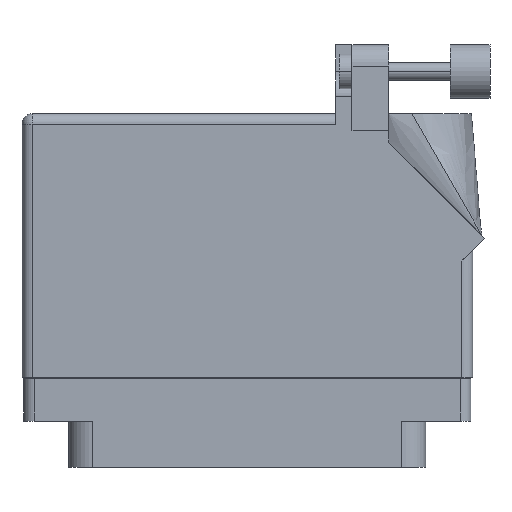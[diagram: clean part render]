
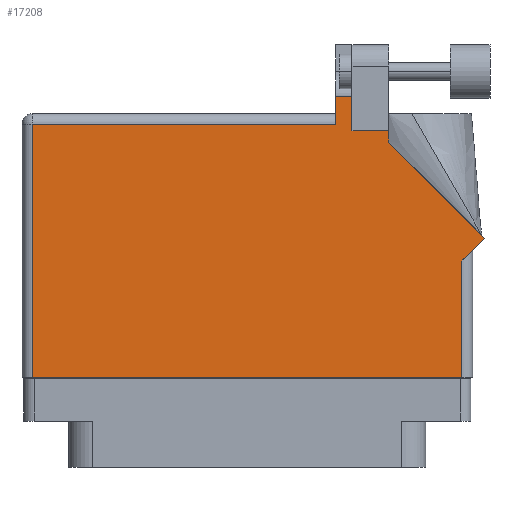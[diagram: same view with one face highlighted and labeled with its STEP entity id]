
A CAD part, front view. The second image highlights one B-rep face of the part: STEP entity #17208.
In plain terms, the highlighted face is planar.
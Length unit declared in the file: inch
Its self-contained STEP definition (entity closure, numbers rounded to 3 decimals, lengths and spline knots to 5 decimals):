
#49 = CARTESIAN_POINT ( 'NONE',  ( 0.513, 1.5315, 0.455 ) ) ;
#221 = VECTOR ( 'NONE', #23083, 39.37008 ) ;
#785 = DIRECTION ( 'NONE',  ( -0.707, 0.707, 0. ) ) ;
#1640 = VERTEX_POINT ( 'NONE', #49 ) ;
#1828 = CARTESIAN_POINT ( 'NONE',  ( 0.82, 1.26442, 0.455 ) ) ;
#2082 = CARTESIAN_POINT ( 'NONE',  ( 0.607, 1.33, 0.455 ) ) ;
#2425 = CARTESIAN_POINT ( 'NONE',  ( 1.244, 0.575, 0.455 ) ) ;
#2976 = DIRECTION ( 'NONE',  ( 0., 1., 0. ) ) ;
#3350 = LINE ( 'NONE', #6694, #26731 ) ;
#3666 = LINE ( 'NONE', #47013, #47791 ) ;
#3968 = CARTESIAN_POINT ( 'NONE',  ( -1.306, -0.1, 0.455 ) ) ;
#4143 = DIRECTION ( 'NONE',  ( 1., 0., 0. ) ) ;
#5109 = DIRECTION ( 'NONE',  ( -1., 0., 0. ) ) ;
#5565 = CARTESIAN_POINT ( 'NONE',  ( 0.82, 1.26442, 0.455 ) ) ;
#5858 = CARTESIAN_POINT ( 'NONE',  ( 0.82, 1.33, 0.455 ) ) ;
#6465 = FACE_OUTER_BOUND ( 'NONE', #18573, .T. ) ;
#6694 = CARTESIAN_POINT ( 'NONE',  ( 0.93777, 1.5315, 0.455 ) ) ;
#7440 = LINE ( 'NONE', #3968, #37716 ) ;
#7619 = LINE ( 'NONE', #27489, #15826 ) ;
#8244 = ORIENTED_EDGE ( 'NONE', *, *, #24293, .T. ) ;
#8708 = DIRECTION ( 'NONE',  ( -1., 0., 0. ) ) ;
#8728 = CARTESIAN_POINT ( 'NONE',  ( -1.306, 1.368, 0.455 ) ) ;
#8995 = LINE ( 'NONE', #29509, #38632 ) ;
#9970 = VERTEX_POINT ( 'NONE', #2425 ) ;
#10563 = VERTEX_POINT ( 'NONE', #39279 ) ;
#10873 = AXIS2_PLACEMENT_3D ( 'NONE', #33602, #33244, #8708 ) ;
#11435 = VERTEX_POINT ( 'NONE', #23367 ) ;
#11550 = DIRECTION ( 'NONE',  ( 0., -1., 0. ) ) ;
#12171 = LINE ( 'NONE', #31360, #221 ) ;
#12985 = VECTOR ( 'NONE', #41783, 39.37008 ) ;
#14093 = EDGE_CURVE ( 'NONE', #51600, #27255, #48488, .T. ) ;
#14761 = EDGE_CURVE ( 'NONE', #37501, #10563, #7440, .T. ) ;
#15752 = CARTESIAN_POINT ( 'NONE',  ( -1.244, -0.1, 0.455 ) ) ;
#15826 = VECTOR ( 'NONE', #2976, 39.37008 ) ;
#17208 = ADVANCED_FACE ( 'NONE', ( #6465 ), #21335, .F. ) ;
#18041 = DIRECTION ( 'NONE',  ( 0., 1., 0. ) ) ;
#18573 = EDGE_LOOP ( 'NONE', ( #34944, #49988, #47823, #34438, #8244, #42310, #28356, #40156, #36596, #33503, #45584 ) ) ;
#18603 = CARTESIAN_POINT ( 'NONE',  ( -1.244, 1.368, 0.455 ) ) ;
#21335 = PLANE ( 'NONE',  #10873 ) ;
#22110 = EDGE_CURVE ( 'NONE', #22245, #1640, #3350, .T. ) ;
#22241 = VECTOR ( 'NONE', #47066, 39.37008 ) ;
#22245 = VERTEX_POINT ( 'NONE', #40136 ) ;
#22596 = LINE ( 'NONE', #43610, #27086 ) ;
#23083 = DIRECTION ( 'NONE',  ( 0.707, 0.707, 0. ) ) ;
#23367 = CARTESIAN_POINT ( 'NONE',  ( 0.513, 1.368, 0.455 ) ) ;
#23704 = LINE ( 'NONE', #5858, #12985 ) ;
#24293 = EDGE_CURVE ( 'NONE', #24915, #37501, #22596, .T. ) ;
#24915 = VERTEX_POINT ( 'NONE', #18603 ) ;
#26731 = VECTOR ( 'NONE', #5109, 39.37008 ) ;
#27063 = VECTOR ( 'NONE', #18041, 39.37008 ) ;
#27086 = VECTOR ( 'NONE', #11550, 39.37008 ) ;
#27255 = VERTEX_POINT ( 'NONE', #47784 ) ;
#27489 = CARTESIAN_POINT ( 'NONE',  ( 0.607, 1.33, 0.455 ) ) ;
#27803 = EDGE_CURVE ( 'NONE', #10563, #9970, #33027, .T. ) ;
#28356 = ORIENTED_EDGE ( 'NONE', *, *, #27803, .T. ) ;
#28566 = EDGE_CURVE ( 'NONE', #11435, #24915, #51197, .T. ) ;
#29267 = EDGE_CURVE ( 'NONE', #41453, #22245, #7619, .T. ) ;
#29509 = CARTESIAN_POINT ( 'NONE',  ( 1.37671, 0.70771, 0.455 ) ) ;
#31321 = DIRECTION ( 'NONE',  ( 0., -1., 0. ) ) ;
#31360 = CARTESIAN_POINT ( 'NONE',  ( 1.306, 0.637, 0.455 ) ) ;
#33027 = LINE ( 'NONE', #41603, #22241 ) ;
#33244 = DIRECTION ( 'NONE',  ( 0., 0., -1. ) ) ;
#33503 = ORIENTED_EDGE ( 'NONE', *, *, #14093, .T. ) ;
#33602 = CARTESIAN_POINT ( 'NONE',  ( -1.306, 1.43, 0.455 ) ) ;
#34438 = ORIENTED_EDGE ( 'NONE', *, *, #28566, .T. ) ;
#34944 = ORIENTED_EDGE ( 'NONE', *, *, #29267, .T. ) ;
#36328 = VERTEX_POINT ( 'NONE', #46859 ) ;
#36596 = ORIENTED_EDGE ( 'NONE', *, *, #37294, .T. ) ;
#37294 = EDGE_CURVE ( 'NONE', #36328, #51600, #8995, .T. ) ;
#37501 = VERTEX_POINT ( 'NONE', #15752 ) ;
#37716 = VECTOR ( 'NONE', #4143, 39.37008 ) ;
#38632 = VECTOR ( 'NONE', #785, 39.37008 ) ;
#39279 = CARTESIAN_POINT ( 'NONE',  ( 1.244, -0.1, 0.455 ) ) ;
#40136 = CARTESIAN_POINT ( 'NONE',  ( 0.607, 1.5315, 0.455 ) ) ;
#40156 = ORIENTED_EDGE ( 'NONE', *, *, #44841, .T. ) ;
#40504 = VECTOR ( 'NONE', #48213, 39.37008 ) ;
#41453 = VERTEX_POINT ( 'NONE', #2082 ) ;
#41603 = CARTESIAN_POINT ( 'NONE',  ( 1.244, 0.637, 0.455 ) ) ;
#41783 = DIRECTION ( 'NONE',  ( -1., 0., 0. ) ) ;
#42310 = ORIENTED_EDGE ( 'NONE', *, *, #14761, .T. ) ;
#43610 = CARTESIAN_POINT ( 'NONE',  ( -1.244, -0.1, 0.455 ) ) ;
#44841 = EDGE_CURVE ( 'NONE', #9970, #36328, #12171, .T. ) ;
#45584 = ORIENTED_EDGE ( 'NONE', *, *, #49491, .T. ) ;
#46859 = CARTESIAN_POINT ( 'NONE',  ( 1.37671, 0.70771, 0.455 ) ) ;
#47013 = CARTESIAN_POINT ( 'NONE',  ( 0.513, 1.43, 0.455 ) ) ;
#47066 = DIRECTION ( 'NONE',  ( 0., 1., 0. ) ) ;
#47784 = CARTESIAN_POINT ( 'NONE',  ( 0.82, 1.33, 0.455 ) ) ;
#47791 = VECTOR ( 'NONE', #31321, 39.37008 ) ;
#47823 = ORIENTED_EDGE ( 'NONE', *, *, #48139, .T. ) ;
#48139 = EDGE_CURVE ( 'NONE', #1640, #11435, #3666, .T. ) ;
#48213 = DIRECTION ( 'NONE',  ( -1., 0., 0. ) ) ;
#48488 = LINE ( 'NONE', #1828, #27063 ) ;
#49491 = EDGE_CURVE ( 'NONE', #27255, #41453, #23704, .T. ) ;
#49988 = ORIENTED_EDGE ( 'NONE', *, *, #22110, .T. ) ;
#51197 = LINE ( 'NONE', #8728, #40504 ) ;
#51600 = VERTEX_POINT ( 'NONE', #5565 ) ;
